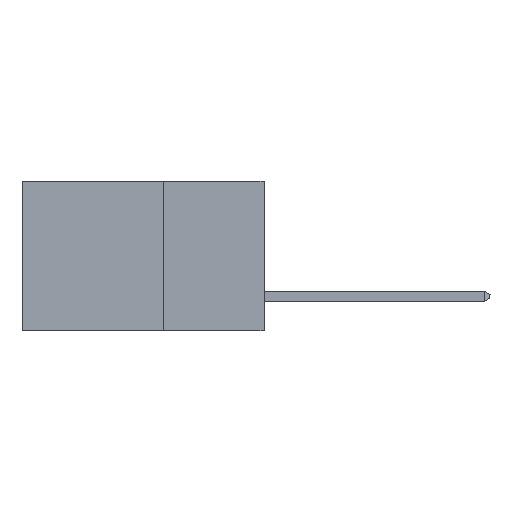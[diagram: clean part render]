
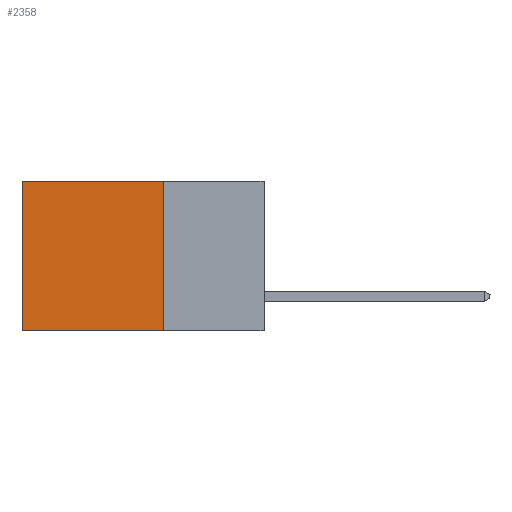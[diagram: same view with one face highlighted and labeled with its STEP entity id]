
A CAD part, left-side view. The second image highlights one B-rep face of the part: STEP entity #2358.
In plain terms, the highlighted planar face has unit normal (-1, 0, 0).
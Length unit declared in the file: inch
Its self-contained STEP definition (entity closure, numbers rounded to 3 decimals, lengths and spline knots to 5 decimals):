
#482 = EDGE_CURVE ( 'NONE', #7249, #1367, #7415, .T. ) ;
#1342 = CARTESIAN_POINT ( 'NONE',  ( 0.2615, 0.25, -0.37 ) ) ;
#1367 = VERTEX_POINT ( 'NONE', #5469 ) ;
#1442 = EDGE_LOOP ( 'NONE', ( #4831, #13625, #4671, #2256 ) ) ;
#1913 = CARTESIAN_POINT ( 'NONE',  ( 0.2615, 0.25, 0. ) ) ;
#2256 = ORIENTED_EDGE ( 'NONE', *, *, #9114, .T. ) ;
#2305 = VECTOR ( 'NONE', #11131, 39.37008 ) ;
#2358 = ADVANCED_FACE ( 'NONE', ( #4358 ), #13106, .F. ) ;
#3299 = CARTESIAN_POINT ( 'NONE',  ( 0.2615, 0.25, -0.37 ) ) ;
#3670 = VECTOR ( 'NONE', #6179, 39.37008 ) ;
#4358 = FACE_OUTER_BOUND ( 'NONE', #1442, .T. ) ;
#4671 = ORIENTED_EDGE ( 'NONE', *, *, #10795, .F. ) ;
#4831 = ORIENTED_EDGE ( 'NONE', *, *, #8137, .T. ) ;
#4934 = CARTESIAN_POINT ( 'NONE',  ( 0.2615, 0.25, -0.37 ) ) ;
#5173 = LINE ( 'NONE', #6185, #9335 ) ;
#5192 = DIRECTION ( 'NONE',  ( 0., 1., 0. ) ) ;
#5469 = CARTESIAN_POINT ( 'NONE',  ( 0.2615, 0.6, -0.37 ) ) ;
#6179 = DIRECTION ( 'NONE',  ( 0., 0., -1. ) ) ;
#6185 = CARTESIAN_POINT ( 'NONE',  ( 0.2615, 0.25, 0. ) ) ;
#6445 = DIRECTION ( 'NONE',  ( 0., 0., -1. ) ) ;
#6987 = CARTESIAN_POINT ( 'NONE',  ( 0.2615, 0.6, 0. ) ) ;
#7249 = VERTEX_POINT ( 'NONE', #4934 ) ;
#7415 = LINE ( 'NONE', #13646, #13696 ) ;
#7437 = AXIS2_PLACEMENT_3D ( 'NONE', #3299, #9668, #6445 ) ;
#8137 = EDGE_CURVE ( 'NONE', #12170, #1367, #11877, .T. ) ;
#9114 = EDGE_CURVE ( 'NONE', #11957, #12170, #5173, .T. ) ;
#9335 = VECTOR ( 'NONE', #10321, 39.37008 ) ;
#9384 = CARTESIAN_POINT ( 'NONE',  ( 0.2615, 0.6, -0.37 ) ) ;
#9668 = DIRECTION ( 'NONE',  ( 1., 0., 0. ) ) ;
#10321 = DIRECTION ( 'NONE',  ( 0., 1., 0. ) ) ;
#10795 = EDGE_CURVE ( 'NONE', #11957, #7249, #12212, .T. ) ;
#11131 = DIRECTION ( 'NONE',  ( 0., 0., -1. ) ) ;
#11877 = LINE ( 'NONE', #9384, #3670 ) ;
#11957 = VERTEX_POINT ( 'NONE', #1913 ) ;
#12170 = VERTEX_POINT ( 'NONE', #6987 ) ;
#12212 = LINE ( 'NONE', #1342, #2305 ) ;
#13106 = PLANE ( 'NONE',  #7437 ) ;
#13625 = ORIENTED_EDGE ( 'NONE', *, *, #482, .F. ) ;
#13646 = CARTESIAN_POINT ( 'NONE',  ( 0.2615, 0.25, -0.37 ) ) ;
#13696 = VECTOR ( 'NONE', #5192, 39.37008 ) ;
